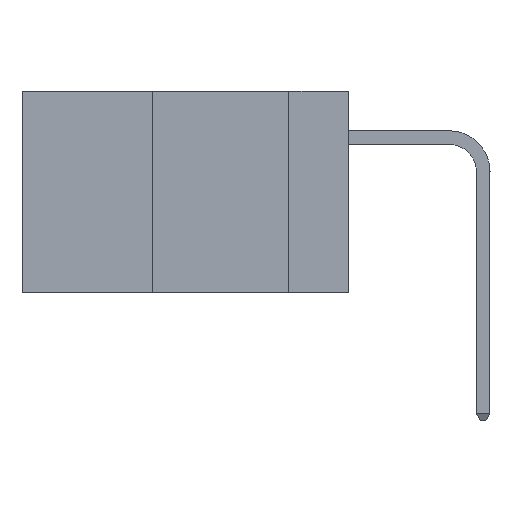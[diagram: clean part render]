
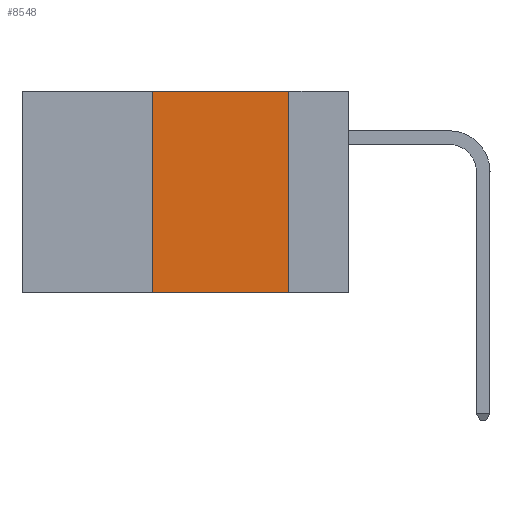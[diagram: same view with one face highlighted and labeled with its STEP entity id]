
A CAD part, left-side view. The second image highlights one B-rep face of the part: STEP entity #8548.
In plain terms, the highlighted planar face has unit normal (-1, 0, 0).
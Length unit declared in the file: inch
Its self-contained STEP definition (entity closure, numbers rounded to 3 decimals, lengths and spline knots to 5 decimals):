
#142 = DIRECTION ( 'NONE',  ( 0., -1., 0. ) ) ;
#642 = CARTESIAN_POINT ( 'NONE',  ( 0., 0.11, -0.37 ) ) ;
#719 = CARTESIAN_POINT ( 'NONE',  ( 0., 0.11, 0. ) ) ;
#1181 = VERTEX_POINT ( 'NONE', #41410 ) ;
#4406 = CARTESIAN_POINT ( 'NONE',  ( 0., 0.36, 0. ) ) ;
#6602 = LINE ( 'NONE', #24484, #34245 ) ;
#6934 = VECTOR ( 'NONE', #7979, 39.37008 ) ;
#6974 = DIRECTION ( 'NONE',  ( 0., -1., 0. ) ) ;
#7247 = ORIENTED_EDGE ( 'NONE', *, *, #9670, .F. ) ;
#7979 = DIRECTION ( 'NONE',  ( 0., 0., 1. ) ) ;
#8548 = ADVANCED_FACE ( 'NONE', ( #28612 ), #19264, .F. ) ;
#9670 = EDGE_CURVE ( 'NONE', #1181, #38129, #11422, .T. ) ;
#10553 = CARTESIAN_POINT ( 'NONE',  ( 0., 0.6, 0. ) ) ;
#11422 = LINE ( 'NONE', #10553, #37561 ) ;
#12827 = DIRECTION ( 'NONE',  ( 0., 0., -1. ) ) ;
#16179 = EDGE_LOOP ( 'NONE', ( #22151, #7247, #31349, #23823 ) ) ;
#17578 = VECTOR ( 'NONE', #32414, 39.37008 ) ;
#18552 = VERTEX_POINT ( 'NONE', #642 ) ;
#19264 = PLANE ( 'NONE',  #42526 ) ;
#19744 = LINE ( 'NONE', #4406, #6934 ) ;
#22151 = ORIENTED_EDGE ( 'NONE', *, *, #36538, .F. ) ;
#22689 = DIRECTION ( 'NONE',  ( 1., 0., 0. ) ) ;
#23823 = ORIENTED_EDGE ( 'NONE', *, *, #35148, .T. ) ;
#24484 = CARTESIAN_POINT ( 'NONE',  ( 0., 0.6, -0.37 ) ) ;
#28612 = FACE_OUTER_BOUND ( 'NONE', #16179, .T. ) ;
#28997 = CARTESIAN_POINT ( 'NONE',  ( 0., 0.36, -0.37 ) ) ;
#29843 = CARTESIAN_POINT ( 'NONE',  ( 0., 0.6, 0. ) ) ;
#31349 = ORIENTED_EDGE ( 'NONE', *, *, #31455, .F. ) ;
#31455 = EDGE_CURVE ( 'NONE', #36629, #1181, #19744, .T. ) ;
#32414 = DIRECTION ( 'NONE',  ( 0., 0., -1. ) ) ;
#34245 = VECTOR ( 'NONE', #142, 39.37008 ) ;
#34606 = LINE ( 'NONE', #38827, #17578 ) ;
#35148 = EDGE_CURVE ( 'NONE', #36629, #18552, #6602, .T. ) ;
#36538 = EDGE_CURVE ( 'NONE', #38129, #18552, #34606, .T. ) ;
#36629 = VERTEX_POINT ( 'NONE', #28997 ) ;
#37561 = VECTOR ( 'NONE', #6974, 39.37008 ) ;
#38129 = VERTEX_POINT ( 'NONE', #719 ) ;
#38827 = CARTESIAN_POINT ( 'NONE',  ( 0., 0.11, 0. ) ) ;
#41410 = CARTESIAN_POINT ( 'NONE',  ( 0., 0.36, 0. ) ) ;
#42526 = AXIS2_PLACEMENT_3D ( 'NONE', #29843, #22689, #12827 ) ;
